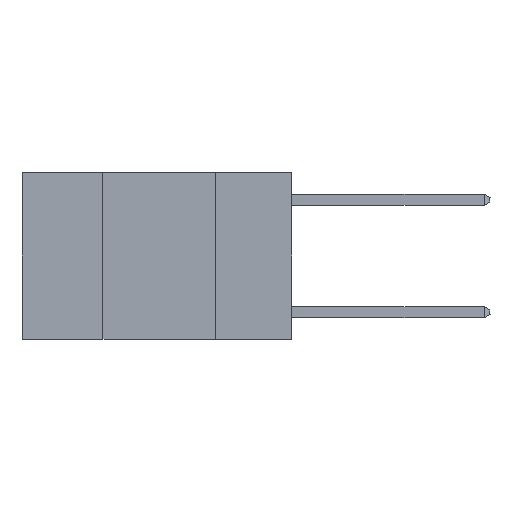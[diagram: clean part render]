
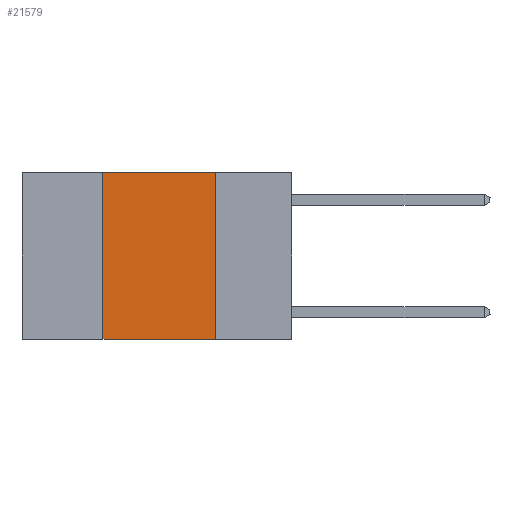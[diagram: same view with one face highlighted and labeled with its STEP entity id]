
A CAD part, left-side view. The second image highlights one B-rep face of the part: STEP entity #21579.
In plain terms, the highlighted planar face has unit normal (-1, 0, 0).
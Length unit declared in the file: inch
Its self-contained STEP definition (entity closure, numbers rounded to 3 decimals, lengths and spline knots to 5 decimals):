
#9 = EDGE_CURVE ( 'NONE', #10447, #6180, #22225, .T. ) ;
#179 = CARTESIAN_POINT ( 'NONE',  ( 0., 0.17, 0. ) ) ;
#360 = EDGE_LOOP ( 'NONE', ( #19311, #22765, #3444, #12204 ) ) ;
#3342 = DIRECTION ( 'NONE',  ( 1., 0., 0. ) ) ;
#3444 = ORIENTED_EDGE ( 'NONE', *, *, #18302, .F. ) ;
#4174 = DIRECTION ( 'NONE',  ( 0., -1., 0. ) ) ;
#4338 = DIRECTION ( 'NONE',  ( 0., -1., 0. ) ) ;
#4669 = EDGE_CURVE ( 'NONE', #15169, #10942, #20615, .T. ) ;
#5137 = PLANE ( 'NONE',  #19501 ) ;
#5150 = VECTOR ( 'NONE', #4338, 39.37008 ) ;
#5915 = DIRECTION ( 'NONE',  ( 0., 0., -1. ) ) ;
#5977 = CARTESIAN_POINT ( 'NONE',  ( 0., 0.42, 0. ) ) ;
#6180 = VERTEX_POINT ( 'NONE', #179 ) ;
#7689 = LINE ( 'NONE', #14831, #9191 ) ;
#8014 = VECTOR ( 'NONE', #4174, 39.37008 ) ;
#8288 = CARTESIAN_POINT ( 'NONE',  ( 0., 0.6, 0. ) ) ;
#9191 = VECTOR ( 'NONE', #5915, 39.37008 ) ;
#10338 = VECTOR ( 'NONE', #20463, 39.37008 ) ;
#10447 = VERTEX_POINT ( 'NONE', #19909 ) ;
#10574 = DIRECTION ( 'NONE',  ( 0., 0., -1. ) ) ;
#10942 = VERTEX_POINT ( 'NONE', #11312 ) ;
#11312 = CARTESIAN_POINT ( 'NONE',  ( 0., 0.17, -0.37 ) ) ;
#12204 = ORIENTED_EDGE ( 'NONE', *, *, #4669, .T. ) ;
#14164 = FACE_OUTER_BOUND ( 'NONE', #360, .T. ) ;
#14831 = CARTESIAN_POINT ( 'NONE',  ( 0., 0.17, 0. ) ) ;
#15169 = VERTEX_POINT ( 'NONE', #20825 ) ;
#16665 = LINE ( 'NONE', #5977, #10338 ) ;
#18302 = EDGE_CURVE ( 'NONE', #15169, #10447, #16665, .T. ) ;
#19287 = EDGE_CURVE ( 'NONE', #6180, #10942, #7689, .T. ) ;
#19311 = ORIENTED_EDGE ( 'NONE', *, *, #19287, .F. ) ;
#19501 = AXIS2_PLACEMENT_3D ( 'NONE', #19613, #3342, #10574 ) ;
#19613 = CARTESIAN_POINT ( 'NONE',  ( 0., 0.6, 0. ) ) ;
#19909 = CARTESIAN_POINT ( 'NONE',  ( 0., 0.42, 0. ) ) ;
#20463 = DIRECTION ( 'NONE',  ( 0., 0., 1. ) ) ;
#20615 = LINE ( 'NONE', #22641, #5150 ) ;
#20825 = CARTESIAN_POINT ( 'NONE',  ( 0., 0.42, -0.37 ) ) ;
#21579 = ADVANCED_FACE ( 'NONE', ( #14164 ), #5137, .F. ) ;
#22225 = LINE ( 'NONE', #8288, #8014 ) ;
#22641 = CARTESIAN_POINT ( 'NONE',  ( 0., 0.6, -0.37 ) ) ;
#22765 = ORIENTED_EDGE ( 'NONE', *, *, #9, .F. ) ;
